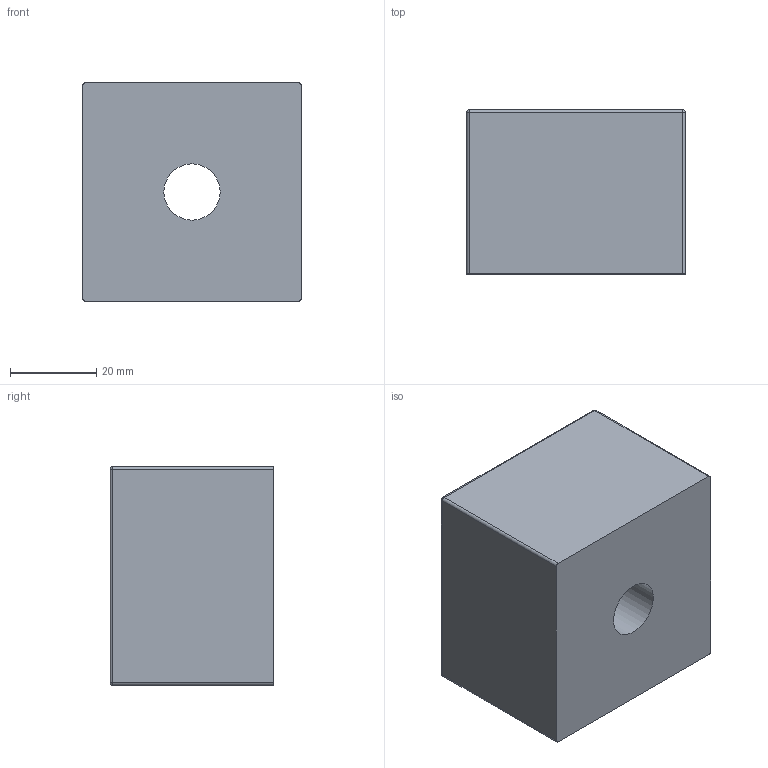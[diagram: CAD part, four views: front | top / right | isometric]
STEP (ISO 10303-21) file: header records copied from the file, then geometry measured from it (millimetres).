
FILE_DESCRIPTION(/* description */ (''),/* implementation_level */ '2;1');
FILE_NAME(/* name */ 'Jig 3.stp',/* time_stamp */ '2019-03-23T15:16:38-05:00',/* author */ ('johne'),/* organization */ (''),/* preprocessor_version */ 'ST-DEVELOPER v16.13',/* originating_system */ 'Autodesk Inventor 2018',/* authorisation */ '');
FILE_SCHEMA (('AUTOMOTIVE_DESIGN { 1 0 10303 214 3 1 1 }'));
Length unit declared in the file: inch
Products named in the file (1): Jig 3
Bounding box: 50.8 x 38.1 x 50.8 mm (x, y, z)
Volume: 85328.7 mm3; surface area: 15116.3 mm2
Topology: 1 solids, 1 shells, 72 faces, 180 edges, 112 vertices
Faces by surface type: plane 24, cylinder 21, bspline 19, sphere 4, torus 4
Full cylindrical faces by diameter (mm): 13.081 x1
Entity records: 2338 total; most frequent: CARTESIAN_POINT 705, ORIENTED_EDGE 358, DIRECTION 275, EDGE_CURVE 179, VERTEX_POINT 112, LINE 99, VECTOR 99, AXIS2_PLACEMENT_3D 88
